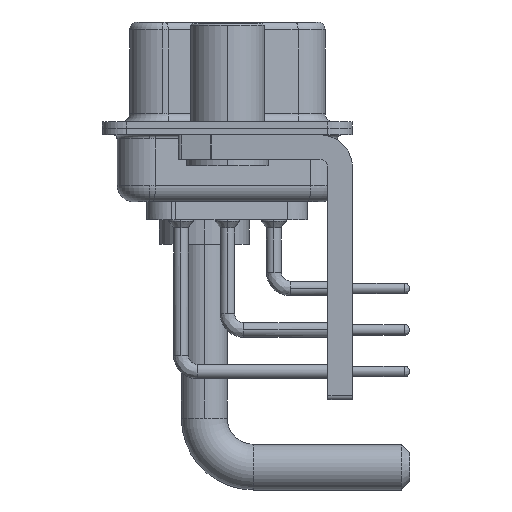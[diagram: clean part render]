
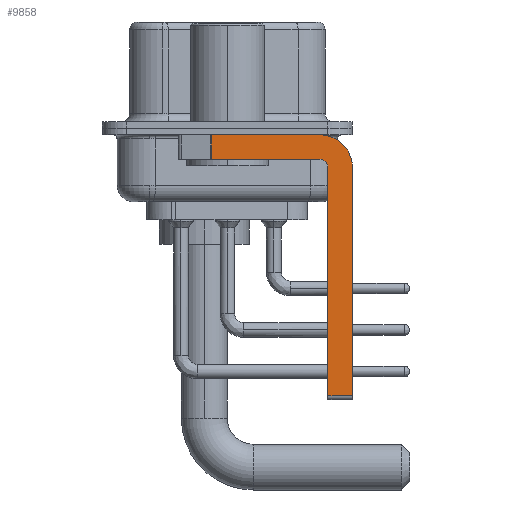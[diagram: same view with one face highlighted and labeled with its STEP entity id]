
A CAD part, left-side view. The second image highlights one B-rep face of the part: STEP entity #9858.
In plain terms, the highlighted planar face has unit normal (-1, 0, 0).
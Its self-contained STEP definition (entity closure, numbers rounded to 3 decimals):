
#1176 = VECTOR ( 'NONE', #21413, 1000. ) ;
#1303 = ORIENTED_EDGE ( 'NONE', *, *, #5314, .F. ) ;
#1331 = CARTESIAN_POINT ( 'NONE',  ( -2.9, -5.65, -16.35 ) ) ;
#1753 = CARTESIAN_POINT ( 'NONE',  ( -2.9, -5.65, -2.4 ) ) ;
#2404 = LINE ( 'NONE', #14364, #1176 ) ;
#2445 = CARTESIAN_POINT ( 'NONE',  ( -2.9, -5.65, -1.9 ) ) ;
#4042 = VERTEX_POINT ( 'NONE', #35532 ) ;
#4169 = ORIENTED_EDGE ( 'NONE', *, *, #35943, .F. ) ;
#4729 = AXIS2_PLACEMENT_3D ( 'NONE', #21870, #18909, #37330 ) ;
#4844 = ORIENTED_EDGE ( 'NONE', *, *, #36095, .F. ) ;
#4950 = CARTESIAN_POINT ( 'NONE',  ( -2.9, -5.65, -2.4 ) ) ;
#5314 = EDGE_CURVE ( 'NONE', #37101, #21815, #2404, .T. ) ;
#5962 = DIRECTION ( 'NONE',  ( 0., 1., 0. ) ) ;
#6409 = VECTOR ( 'NONE', #32252, 1000. ) ;
#6530 = CARTESIAN_POINT ( 'NONE',  ( -2.9, -5.65, -0.4 ) ) ;
#6536 = VERTEX_POINT ( 'NONE', #34620 ) ;
#7860 = CIRCLE ( 'NONE', #24128, 0.5 ) ;
#7889 = PLANE ( 'NONE',  #20664 ) ;
#8218 = CARTESIAN_POINT ( 'NONE',  ( -2.9, 0.978, -1.9 ) ) ;
#8397 = DIRECTION ( 'NONE',  ( 0., 0., -1. ) ) ;
#8398 = EDGE_CURVE ( 'NONE', #6536, #18341, #25580, .T. ) ;
#9858 = ADVANCED_FACE ( 'NONE', ( #34736 ), #7889, .F. ) ;
#10862 = EDGE_CURVE ( 'NONE', #6536, #11082, #13512, .T. ) ;
#11082 = VERTEX_POINT ( 'NONE', #20535 ) ;
#11336 = VECTOR ( 'NONE', #5962, 1000. ) ;
#12005 = EDGE_CURVE ( 'NONE', #4042, #38647, #37932, .T. ) ;
#13340 = CARTESIAN_POINT ( 'NONE',  ( -2.9, -7.65, -2.4 ) ) ;
#13512 = LINE ( 'NONE', #1331, #15619 ) ;
#14364 = CARTESIAN_POINT ( 'NONE',  ( -2.9, 3., -0.4 ) ) ;
#14474 = LINE ( 'NONE', #20938, #33258 ) ;
#15619 = VECTOR ( 'NONE', #28991, 1000. ) ;
#16764 = EDGE_LOOP ( 'NONE', ( #1303, #30084, #36102, #4169, #34972, #20524, #23633, #4844 ) ) ;
#16765 = CARTESIAN_POINT ( 'NONE',  ( -2.9, -7.65, -2.4 ) ) ;
#16898 = DIRECTION ( 'NONE',  ( 1., 0., 0. ) ) ;
#18341 = VERTEX_POINT ( 'NONE', #30879 ) ;
#18909 = DIRECTION ( 'NONE',  ( 1., 0., 0. ) ) ;
#20524 = ORIENTED_EDGE ( 'NONE', *, *, #10862, .T. ) ;
#20535 = CARTESIAN_POINT ( 'NONE',  ( -2.9, -7.65, -16.35 ) ) ;
#20664 = AXIS2_PLACEMENT_3D ( 'NONE', #4950, #16898, #28894 ) ;
#20697 = DIRECTION ( 'NONE',  ( -1., 0., 0. ) ) ;
#20938 = CARTESIAN_POINT ( 'NONE',  ( -2.9, 0.978, -1.9 ) ) ;
#21413 = DIRECTION ( 'NONE',  ( 0., -1., 0. ) ) ;
#21678 = DIRECTION ( 'NONE',  ( 0., 0., 1. ) ) ;
#21815 = VERTEX_POINT ( 'NONE', #6530 ) ;
#21870 = CARTESIAN_POINT ( 'NONE',  ( -2.9, -5.65, -2.4 ) ) ;
#22853 = LINE ( 'NONE', #16765, #6409 ) ;
#23633 = ORIENTED_EDGE ( 'NONE', *, *, #24109, .F. ) ;
#24109 = EDGE_CURVE ( 'NONE', #30304, #11082, #22853, .T. ) ;
#24128 = AXIS2_PLACEMENT_3D ( 'NONE', #1753, #20697, #21678 ) ;
#25396 = DIRECTION ( 'NONE',  ( 0., 0., 1. ) ) ;
#25399 = CIRCLE ( 'NONE', #4729, 2. ) ;
#25580 = LINE ( 'NONE', #31095, #25601 ) ;
#25601 = VECTOR ( 'NONE', #25396, 1000. ) ;
#28894 = DIRECTION ( 'NONE',  ( 0., 0., -1. ) ) ;
#28991 = DIRECTION ( 'NONE',  ( 0., -1., 0. ) ) ;
#30084 = ORIENTED_EDGE ( 'NONE', *, *, #30596, .T. ) ;
#30304 = VERTEX_POINT ( 'NONE', #13340 ) ;
#30596 = EDGE_CURVE ( 'NONE', #37101, #38647, #14474, .T. ) ;
#30879 = CARTESIAN_POINT ( 'NONE',  ( -2.9, -6.15, -2.4 ) ) ;
#31095 = CARTESIAN_POINT ( 'NONE',  ( -2.9, -6.15, -16.6 ) ) ;
#32252 = DIRECTION ( 'NONE',  ( 0., 0., -1. ) ) ;
#33258 = VECTOR ( 'NONE', #8397, 1000. ) ;
#33708 = CARTESIAN_POINT ( 'NONE',  ( -2.9, 0.978, -0.4 ) ) ;
#34620 = CARTESIAN_POINT ( 'NONE',  ( -2.9, -6.15, -16.35 ) ) ;
#34736 = FACE_OUTER_BOUND ( 'NONE', #16764, .T. ) ;
#34972 = ORIENTED_EDGE ( 'NONE', *, *, #8398, .F. ) ;
#35532 = CARTESIAN_POINT ( 'NONE',  ( -2.9, -5.65, -1.9 ) ) ;
#35943 = EDGE_CURVE ( 'NONE', #18341, #4042, #7860, .T. ) ;
#36095 = EDGE_CURVE ( 'NONE', #21815, #30304, #25399, .T. ) ;
#36102 = ORIENTED_EDGE ( 'NONE', *, *, #12005, .F. ) ;
#37101 = VERTEX_POINT ( 'NONE', #33708 ) ;
#37330 = DIRECTION ( 'NONE',  ( 0., 0., -1. ) ) ;
#37932 = LINE ( 'NONE', #2445, #11336 ) ;
#38647 = VERTEX_POINT ( 'NONE', #8218 ) ;
